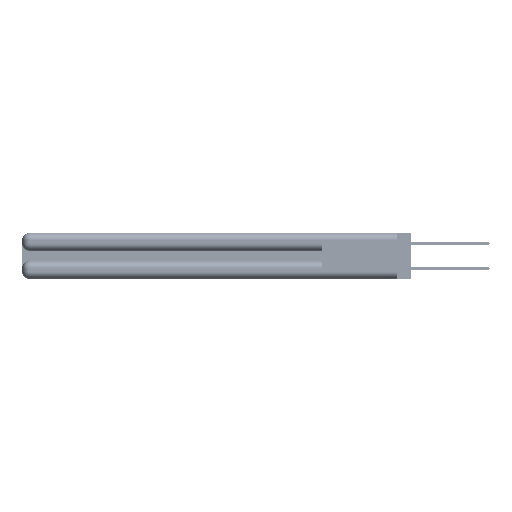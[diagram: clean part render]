
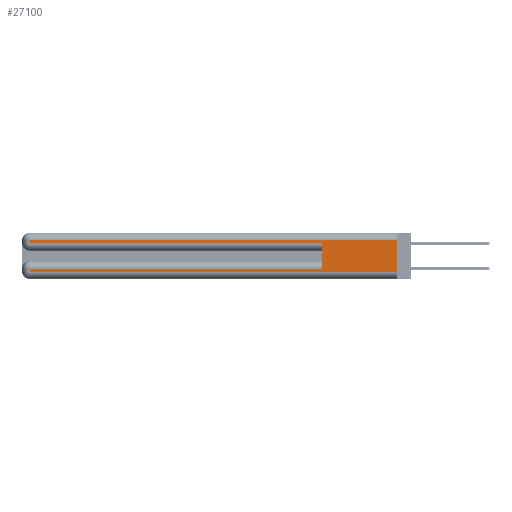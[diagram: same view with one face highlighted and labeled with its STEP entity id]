
A CAD part, left-side view. The second image highlights one B-rep face of the part: STEP entity #27100.
In plain terms, the highlighted planar face has unit normal (-1, 0, 0).
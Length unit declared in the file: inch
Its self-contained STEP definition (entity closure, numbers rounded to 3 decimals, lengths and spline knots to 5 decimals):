
#679 = DIRECTION ( 'NONE',  ( 0., 0., -1. ) ) ;
#1051 = CARTESIAN_POINT ( 'NONE',  ( 0., 0., 0.37 ) ) ;
#1599 = DIRECTION ( 'NONE',  ( 0., 1., 0. ) ) ;
#2333 = EDGE_CURVE ( 'NONE', #38779, #36513, #11206, .T. ) ;
#2659 = CARTESIAN_POINT ( 'NONE',  ( 0., 0., 0.37 ) ) ;
#5455 = VECTOR ( 'NONE', #26036, 39.37008 ) ;
#5643 = DIRECTION ( 'NONE',  ( 0., -1., 0. ) ) ;
#7857 = EDGE_CURVE ( 'NONE', #19816, #23463, #11087, .T. ) ;
#8332 = DIRECTION ( 'NONE',  ( 0., 0., -1. ) ) ;
#9306 = AXIS2_PLACEMENT_3D ( 'NONE', #2659, #15981, #46846 ) ;
#10327 = VERTEX_POINT ( 'NONE', #55011 ) ;
#10476 = CARTESIAN_POINT ( 'NONE',  ( 0., 0., 0.31 ) ) ;
#10862 = LINE ( 'NONE', #1051, #21196 ) ;
#11087 = LINE ( 'NONE', #21451, #34559 ) ;
#11206 = LINE ( 'NONE', #34781, #46413 ) ;
#11874 = ORIENTED_EDGE ( 'NONE', *, *, #15792, .T. ) ;
#12289 = CARTESIAN_POINT ( 'NONE',  ( 0., 0.6, 0.145 ) ) ;
#12804 = VERTEX_POINT ( 'NONE', #47125 ) ;
#13114 = VERTEX_POINT ( 'NONE', #18332 ) ;
#15792 = EDGE_CURVE ( 'NONE', #36513, #13114, #30022, .T. ) ;
#15981 = DIRECTION ( 'NONE',  ( 1., 0., 0. ) ) ;
#18332 = CARTESIAN_POINT ( 'NONE',  ( 0., 0.6, 0.285 ) ) ;
#19816 = VERTEX_POINT ( 'NONE', #31223 ) ;
#21153 = EDGE_LOOP ( 'NONE', ( #25120, #56664, #29850, #11874, #27167, #39511, #24891, #54133 ) ) ;
#21196 = VECTOR ( 'NONE', #49495, 39.37008 ) ;
#21451 = CARTESIAN_POINT ( 'NONE',  ( 0., 0., 0.06 ) ) ;
#22098 = LINE ( 'NONE', #12289, #55974 ) ;
#22112 = EDGE_CURVE ( 'NONE', #12804, #19816, #33833, .T. ) ;
#22657 = CARTESIAN_POINT ( 'NONE',  ( 0., 2.94, 0.37 ) ) ;
#23463 = VERTEX_POINT ( 'NONE', #27261 ) ;
#24891 = ORIENTED_EDGE ( 'NONE', *, *, #22112, .T. ) ;
#25120 = ORIENTED_EDGE ( 'NONE', *, *, #28644, .F. ) ;
#26036 = DIRECTION ( 'NONE',  ( 0., 1., 0. ) ) ;
#26720 = EDGE_CURVE ( 'NONE', #42478, #12804, #40698, .T. ) ;
#27100 = ADVANCED_FACE ( 'NONE', ( #46172 ), #42399, .F. ) ;
#27167 = ORIENTED_EDGE ( 'NONE', *, *, #35123, .F. ) ;
#27261 = CARTESIAN_POINT ( 'NONE',  ( 0., 0., 0.06 ) ) ;
#28644 = EDGE_CURVE ( 'NONE', #10327, #23463, #10862, .T. ) ;
#28654 = VECTOR ( 'NONE', #5643, 39.37008 ) ;
#29850 = ORIENTED_EDGE ( 'NONE', *, *, #2333, .T. ) ;
#30022 = LINE ( 'NONE', #54098, #28654 ) ;
#31223 = CARTESIAN_POINT ( 'NONE',  ( 0., 2.94, 0.06 ) ) ;
#33628 = EDGE_CURVE ( 'NONE', #10327, #38779, #55478, .T. ) ;
#33833 = LINE ( 'NONE', #22657, #44135 ) ;
#34559 = VECTOR ( 'NONE', #47910, 39.37008 ) ;
#34781 = CARTESIAN_POINT ( 'NONE',  ( 0., 2.94, 0.37 ) ) ;
#35123 = EDGE_CURVE ( 'NONE', #42478, #13114, #22098, .T. ) ;
#36449 = CARTESIAN_POINT ( 'NONE',  ( 0., 2.94, 0.31 ) ) ;
#36513 = VERTEX_POINT ( 'NONE', #52094 ) ;
#38755 = DIRECTION ( 'NONE',  ( 0., 0., 1. ) ) ;
#38779 = VERTEX_POINT ( 'NONE', #36449 ) ;
#39511 = ORIENTED_EDGE ( 'NONE', *, *, #26720, .T. ) ;
#40698 = LINE ( 'NONE', #52492, #5455 ) ;
#42399 = PLANE ( 'NONE',  #9306 ) ;
#42478 = VERTEX_POINT ( 'NONE', #49015 ) ;
#43699 = VECTOR ( 'NONE', #1599, 39.37008 ) ;
#44135 = VECTOR ( 'NONE', #679, 39.37008 ) ;
#46172 = FACE_OUTER_BOUND ( 'NONE', #21153, .T. ) ;
#46413 = VECTOR ( 'NONE', #8332, 39.37008 ) ;
#46846 = DIRECTION ( 'NONE',  ( 0., 0., -1. ) ) ;
#47125 = CARTESIAN_POINT ( 'NONE',  ( 0., 2.94, 0.085 ) ) ;
#47910 = DIRECTION ( 'NONE',  ( 0., -1., 0. ) ) ;
#49015 = CARTESIAN_POINT ( 'NONE',  ( 0., 0.6, 0.085 ) ) ;
#49495 = DIRECTION ( 'NONE',  ( 0., 0., -1. ) ) ;
#52094 = CARTESIAN_POINT ( 'NONE',  ( 0., 2.94, 0.285 ) ) ;
#52492 = CARTESIAN_POINT ( 'NONE',  ( 0., 0., 0.085 ) ) ;
#54098 = CARTESIAN_POINT ( 'NONE',  ( 0., 0., 0.285 ) ) ;
#54133 = ORIENTED_EDGE ( 'NONE', *, *, #7857, .T. ) ;
#55011 = CARTESIAN_POINT ( 'NONE',  ( 0., 0., 0.31 ) ) ;
#55478 = LINE ( 'NONE', #10476, #43699 ) ;
#55974 = VECTOR ( 'NONE', #38755, 39.37008 ) ;
#56664 = ORIENTED_EDGE ( 'NONE', *, *, #33628, .T. ) ;
